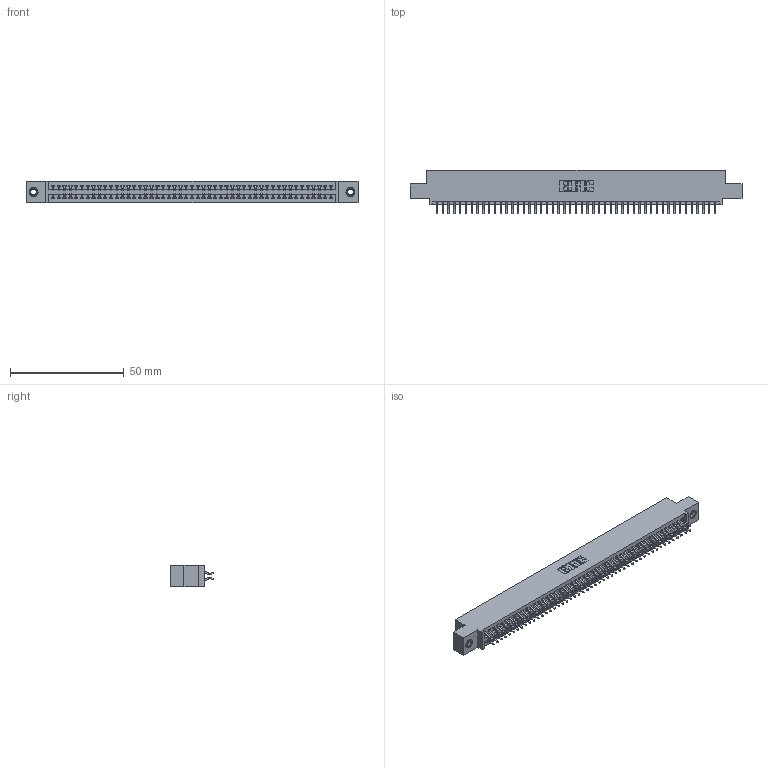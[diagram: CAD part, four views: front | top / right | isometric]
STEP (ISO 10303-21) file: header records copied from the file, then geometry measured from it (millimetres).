
FILE_DESCRIPTION (( 'STEP AP203' ), '1' );
FILE_NAME ('395-098-556-507.STEP', '2019-10-26T13:56:32', ( '' ), ( '' ), 'SwSTEP 2.0', 'SolidWorks 2016', '' );
FILE_SCHEMA (( 'CONFIG_CONTROL_DESIGN' ));
Length unit declared in the file: inch
Products named in the file (4): 345-292-001_556 Tail; 345-250-001_345-250-005-103; 395-098-556-507; 345 Part_0.110 Offset - 0.156 Dia-TI
Assembly tree (101 placements, depth 2):
  395-098-556-507
    345 Part_0.110 Offset - 0.156 Dia-TI
    345-292-001_556 Tail  x98
    345-250-001_345-250-005-103  x2
Bounding box: 145.67 x 19.24 x 9.4 mm (x, y, z)
Volume: 14124.7 mm3; surface area: 21049.1 mm2
Topology: 101 solids, 101 shells, 5678 faces, 16855 edges, 11098 vertices
Faces by surface type: plane 3742, cylinder 1920, cone 12, torus 4
Entity records: 39042 total; most frequent: CARTESIAN_POINT 6535, ORIENTED_EDGE 6450, DIRECTION 5767, EDGE_CURVE 3225, LINE 2869, VECTOR 2869, VERTEX_POINT 2144, AXIS2_PLACEMENT_3D 1449
